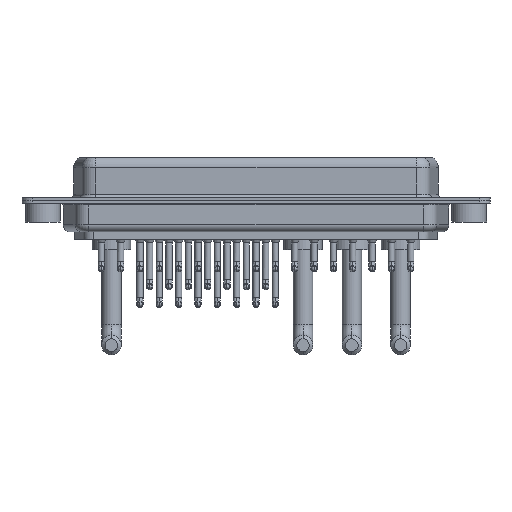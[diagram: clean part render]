
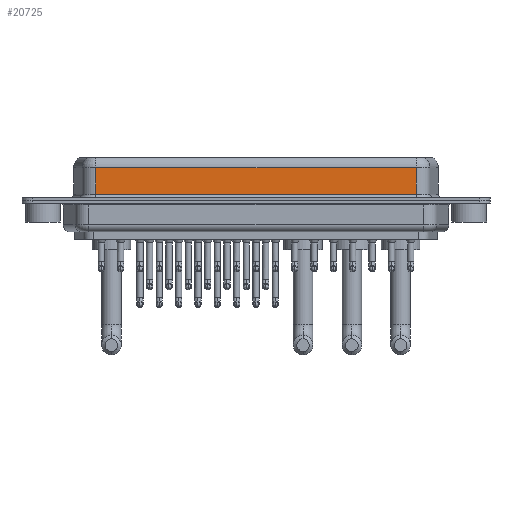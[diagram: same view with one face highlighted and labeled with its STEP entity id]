
A CAD part, front view. The second image highlights one B-rep face of the part: STEP entity #20725.
In plain terms, the highlighted planar face has unit normal (0, -1, 0).
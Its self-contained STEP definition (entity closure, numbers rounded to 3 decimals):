
#390 = LINE ( 'NONE', #7538, #24020 ) ;
#1418 = VECTOR ( 'NONE', #22316, 1000. ) ;
#1640 = DIRECTION ( 'NONE',  ( 0., 1., 0. ) ) ;
#2962 = AXIS2_PLACEMENT_3D ( 'NONE', #22005, #1640, #19767 ) ;
#3777 = CARTESIAN_POINT ( 'NONE',  ( 53.41, -5.375, 0.9 ) ) ;
#7538 = CARTESIAN_POINT ( 'NONE',  ( 53.41, -5.375, 4.65 ) ) ;
#7633 = CARTESIAN_POINT ( 'NONE',  ( 7.59, -5.375, 4.65 ) ) ;
#7661 = EDGE_CURVE ( 'NONE', #19721, #27708, #390, .T. ) ;
#8813 = CARTESIAN_POINT ( 'NONE',  ( 7.59, -5.375, 6.4 ) ) ;
#9482 = DIRECTION ( 'NONE',  ( -1., 0., 0. ) ) ;
#9851 = EDGE_CURVE ( 'NONE', #18156, #26913, #26378, .T. ) ;
#9912 = VECTOR ( 'NONE', #17523, 1000. ) ;
#11743 = ORIENTED_EDGE ( 'NONE', *, *, #7661, .T. ) ;
#12934 = PLANE ( 'NONE',  #2962 ) ;
#13734 = EDGE_LOOP ( 'NONE', ( #28045, #11743, #21169, #15171 ) ) ;
#15171 = ORIENTED_EDGE ( 'NONE', *, *, #9851, .T. ) ;
#17523 = DIRECTION ( 'NONE',  ( 0., 0., -1. ) ) ;
#17833 = EDGE_CURVE ( 'NONE', #19721, #26913, #24362, .T. ) ;
#18156 = VERTEX_POINT ( 'NONE', #23294 ) ;
#19300 = CARTESIAN_POINT ( 'NONE',  ( 53.41, -5.375, 6.4 ) ) ;
#19400 = EDGE_CURVE ( 'NONE', #27708, #18156, #22029, .T. ) ;
#19721 = VERTEX_POINT ( 'NONE', #20305 ) ;
#19767 = DIRECTION ( 'NONE',  ( 0., 0., 1. ) ) ;
#20305 = CARTESIAN_POINT ( 'NONE',  ( 53.41, -5.375, 4.65 ) ) ;
#20725 = ADVANCED_FACE ( 'NONE', ( #24242 ), #12934, .F. ) ;
#21169 = ORIENTED_EDGE ( 'NONE', *, *, #19400, .T. ) ;
#21328 = DIRECTION ( 'NONE',  ( 1., 0., 0. ) ) ;
#22005 = CARTESIAN_POINT ( 'NONE',  ( 53.41, -5.375, 6.4 ) ) ;
#22029 = LINE ( 'NONE', #8813, #1418 ) ;
#22316 = DIRECTION ( 'NONE',  ( 0., 0., -1. ) ) ;
#23294 = CARTESIAN_POINT ( 'NONE',  ( 7.59, -5.375, 0.9 ) ) ;
#24020 = VECTOR ( 'NONE', #9482, 1000. ) ;
#24242 = FACE_OUTER_BOUND ( 'NONE', #13734, .T. ) ;
#24362 = LINE ( 'NONE', #19300, #9912 ) ;
#26378 = LINE ( 'NONE', #26528, #29272 ) ;
#26528 = CARTESIAN_POINT ( 'NONE',  ( 53.41, -5.375, 0.9 ) ) ;
#26913 = VERTEX_POINT ( 'NONE', #3777 ) ;
#27708 = VERTEX_POINT ( 'NONE', #7633 ) ;
#28045 = ORIENTED_EDGE ( 'NONE', *, *, #17833, .F. ) ;
#29272 = VECTOR ( 'NONE', #21328, 1000. ) ;
